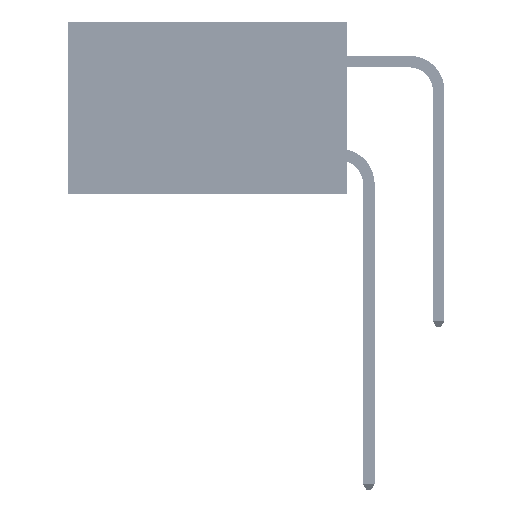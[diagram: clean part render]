
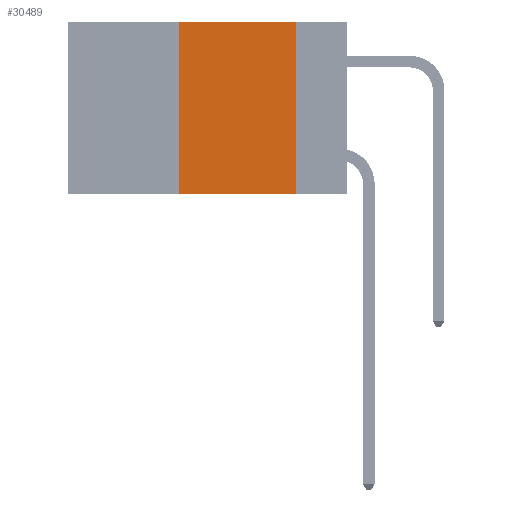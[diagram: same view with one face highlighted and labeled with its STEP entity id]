
A CAD part, left-side view. The second image highlights one B-rep face of the part: STEP entity #30489.
In plain terms, the highlighted planar face has unit normal (-1, 0, 0).
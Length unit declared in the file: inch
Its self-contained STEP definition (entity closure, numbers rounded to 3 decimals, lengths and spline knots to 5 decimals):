
#187 = VERTEX_POINT ( 'NONE', #199 ) ;
#199 = CARTESIAN_POINT ( 'NONE',  ( 0., 0.36, -0.37 ) ) ;
#2281 = CARTESIAN_POINT ( 'NONE',  ( 0., 0.6, 0. ) ) ;
#2739 = PLANE ( 'NONE',  #27813 ) ;
#3128 = ORIENTED_EDGE ( 'NONE', *, *, #16008, .F. ) ;
#3895 = DIRECTION ( 'NONE',  ( 0., 0., -1. ) ) ;
#4263 = CARTESIAN_POINT ( 'NONE',  ( 0., 0.11, -0.37 ) ) ;
#5335 = DIRECTION ( 'NONE',  ( 0., -1., 0. ) ) ;
#7626 = CARTESIAN_POINT ( 'NONE',  ( 0., 0.11, 0. ) ) ;
#7627 = VERTEX_POINT ( 'NONE', #7626 ) ;
#9404 = LINE ( 'NONE', #30080, #32172 ) ;
#10405 = DIRECTION ( 'NONE',  ( 0., -1., 0. ) ) ;
#11706 = VECTOR ( 'NONE', #10405, 39.37008 ) ;
#14232 = LINE ( 'NONE', #44009, #19644 ) ;
#15338 = VECTOR ( 'NONE', #5335, 39.37008 ) ;
#16008 = EDGE_CURVE ( 'NONE', #31710, #7627, #18300, .T. ) ;
#17735 = DIRECTION ( 'NONE',  ( 0., 0., -1. ) ) ;
#18250 = DIRECTION ( 'NONE',  ( 1., 0., 0. ) ) ;
#18300 = LINE ( 'NONE', #2281, #11706 ) ;
#18343 = EDGE_CURVE ( 'NONE', #187, #47569, #26725, .T. ) ;
#19644 = VECTOR ( 'NONE', #40454, 39.37008 ) ;
#26725 = LINE ( 'NONE', #34867, #15338 ) ;
#27813 = AXIS2_PLACEMENT_3D ( 'NONE', #29251, #18250, #17735 ) ;
#29251 = CARTESIAN_POINT ( 'NONE',  ( 0., 0.6, 0. ) ) ;
#29870 = EDGE_LOOP ( 'NONE', ( #37335, #3128, #41903, #31275 ) ) ;
#30080 = CARTESIAN_POINT ( 'NONE',  ( 0., 0.11, 0. ) ) ;
#30489 = ADVANCED_FACE ( 'NONE', ( #46155 ), #2739, .F. ) ;
#31275 = ORIENTED_EDGE ( 'NONE', *, *, #18343, .T. ) ;
#31710 = VERTEX_POINT ( 'NONE', #43582 ) ;
#32172 = VECTOR ( 'NONE', #3895, 39.37008 ) ;
#34867 = CARTESIAN_POINT ( 'NONE',  ( 0., 0.6, -0.37 ) ) ;
#37335 = ORIENTED_EDGE ( 'NONE', *, *, #48276, .F. ) ;
#40454 = DIRECTION ( 'NONE',  ( 0., 0., 1. ) ) ;
#41903 = ORIENTED_EDGE ( 'NONE', *, *, #47832, .F. ) ;
#43582 = CARTESIAN_POINT ( 'NONE',  ( 0., 0.36, 0. ) ) ;
#44009 = CARTESIAN_POINT ( 'NONE',  ( 0., 0.36, 0. ) ) ;
#46155 = FACE_OUTER_BOUND ( 'NONE', #29870, .T. ) ;
#47569 = VERTEX_POINT ( 'NONE', #4263 ) ;
#47832 = EDGE_CURVE ( 'NONE', #187, #31710, #14232, .T. ) ;
#48276 = EDGE_CURVE ( 'NONE', #7627, #47569, #9404, .T. ) ;
